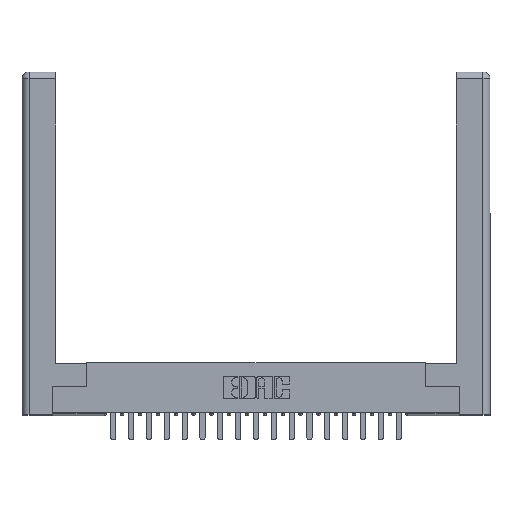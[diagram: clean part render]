
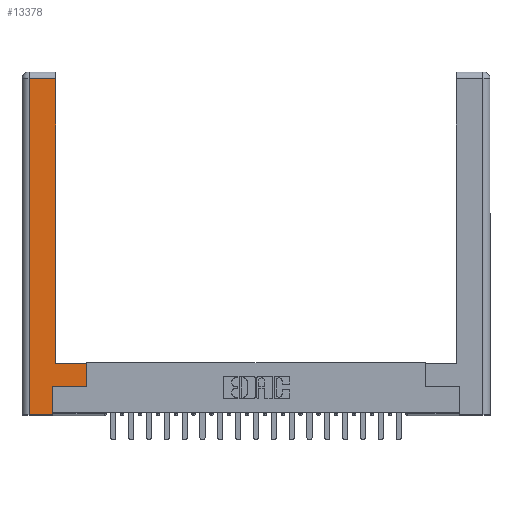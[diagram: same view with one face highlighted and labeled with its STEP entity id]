
A CAD part, top view. The second image highlights one B-rep face of the part: STEP entity #13378.
In plain terms, the highlighted planar face has unit normal (0, 0, 1).
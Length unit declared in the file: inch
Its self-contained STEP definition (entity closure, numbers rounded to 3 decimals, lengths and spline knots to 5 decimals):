
#65 = LINE ( 'NONE', #10941, #19154 ) ;
#107 = VECTOR ( 'NONE', #4367, 39.37008 ) ;
#343 = LINE ( 'NONE', #12468, #22065 ) ;
#572 = DIRECTION ( 'NONE',  ( -1., 0., 0. ) ) ;
#976 = CARTESIAN_POINT ( 'NONE',  ( 0.565, 0.245, 0. ) ) ;
#1050 = ORIENTED_EDGE ( 'NONE', *, *, #21979, .T. ) ;
#1167 = VECTOR ( 'NONE', #1383, 39.37008 ) ;
#1187 = LINE ( 'NONE', #21142, #4962 ) ;
#1383 = DIRECTION ( 'NONE',  ( 1., 0., 0. ) ) ;
#1439 = DIRECTION ( 'NONE',  ( 1., 0., 0. ) ) ;
#1939 = PLANE ( 'NONE',  #17478 ) ;
#2504 = CARTESIAN_POINT ( 'NONE',  ( 0.295, 0.45, 0. ) ) ;
#2881 = LINE ( 'NONE', #6658, #11604 ) ;
#2924 = DIRECTION ( 'NONE',  ( 0., 1., 0. ) ) ;
#3566 = ORIENTED_EDGE ( 'NONE', *, *, #14020, .T. ) ;
#4140 = LINE ( 'NONE', #15375, #20902 ) ;
#4367 = DIRECTION ( 'NONE',  ( 0., 1., 0. ) ) ;
#4962 = VECTOR ( 'NONE', #10049, 39.37008 ) ;
#5675 = VERTEX_POINT ( 'NONE', #2504 ) ;
#6290 = ORIENTED_EDGE ( 'NONE', *, *, #6470, .T. ) ;
#6310 = CARTESIAN_POINT ( 'NONE',  ( 0.295, 3., 0. ) ) ;
#6318 = CARTESIAN_POINT ( 'NONE',  ( 0.295, 2.94, 0. ) ) ;
#6350 = VERTEX_POINT ( 'NONE', #6318 ) ;
#6398 = EDGE_CURVE ( 'NONE', #6350, #15645, #4140, .T. ) ;
#6470 = EDGE_CURVE ( 'NONE', #15645, #20443, #65, .T. ) ;
#6608 = LINE ( 'NONE', #12666, #12117 ) ;
#6658 = CARTESIAN_POINT ( 'NONE',  ( 0.565, 0.45, 0. ) ) ;
#7301 = DIRECTION ( 'NONE',  ( 0., -1., 0. ) ) ;
#8088 = ORIENTED_EDGE ( 'NONE', *, *, #8609, .T. ) ;
#8609 = EDGE_CURVE ( 'NONE', #12126, #16049, #2881, .T. ) ;
#9026 = DIRECTION ( 'NONE',  ( 0., 1., 0. ) ) ;
#9556 = DIRECTION ( 'NONE',  ( 0., 0., -1. ) ) ;
#10049 = DIRECTION ( 'NONE',  ( -1., 0., 0. ) ) ;
#10516 = LINE ( 'NONE', #6310, #107 ) ;
#10620 = CARTESIAN_POINT ( 'NONE',  ( 0.565, 0.245, 0. ) ) ;
#10941 = CARTESIAN_POINT ( 'NONE',  ( 0.0615, 0., 0. ) ) ;
#11268 = DIRECTION ( 'NONE',  ( -1., 0., 0. ) ) ;
#11604 = VECTOR ( 'NONE', #2924, 39.37008 ) ;
#12117 = VECTOR ( 'NONE', #9026, 39.37008 ) ;
#12126 = VERTEX_POINT ( 'NONE', #976 ) ;
#12283 = EDGE_CURVE ( 'NONE', #13593, #12126, #14204, .T. ) ;
#12429 = FACE_OUTER_BOUND ( 'NONE', #15455, .T. ) ;
#12468 = CARTESIAN_POINT ( 'NONE',  ( 0.265, 0., 0. ) ) ;
#12492 = ORIENTED_EDGE ( 'NONE', *, *, #12283, .T. ) ;
#12666 = CARTESIAN_POINT ( 'NONE',  ( 0.265, 0.245, 0. ) ) ;
#13378 = ADVANCED_FACE ( 'NONE', ( #12429 ), #1939, .F. ) ;
#13593 = VERTEX_POINT ( 'NONE', #21556 ) ;
#14020 = EDGE_CURVE ( 'NONE', #23426, #13593, #6608, .T. ) ;
#14204 = LINE ( 'NONE', #10620, #1167 ) ;
#14820 = CARTESIAN_POINT ( 'NONE',  ( 0.565, 0.45, 0. ) ) ;
#14898 = ORIENTED_EDGE ( 'NONE', *, *, #6398, .T. ) ;
#15375 = CARTESIAN_POINT ( 'NONE',  ( 0.0615, 2.94, 0. ) ) ;
#15455 = EDGE_LOOP ( 'NONE', ( #1050, #14898, #6290, #18041, #3566, #12492, #8088, #17053 ) ) ;
#15645 = VERTEX_POINT ( 'NONE', #17046 ) ;
#16049 = VERTEX_POINT ( 'NONE', #14820 ) ;
#16658 = CARTESIAN_POINT ( 'NONE',  ( 0., 0., 0. ) ) ;
#17046 = CARTESIAN_POINT ( 'NONE',  ( 0.0615, 2.94, 0. ) ) ;
#17053 = ORIENTED_EDGE ( 'NONE', *, *, #17248, .T. ) ;
#17130 = EDGE_CURVE ( 'NONE', #20443, #23426, #343, .T. ) ;
#17248 = EDGE_CURVE ( 'NONE', #16049, #5675, #1187, .T. ) ;
#17478 = AXIS2_PLACEMENT_3D ( 'NONE', #16658, #9556, #11268 ) ;
#18041 = ORIENTED_EDGE ( 'NONE', *, *, #17130, .T. ) ;
#19154 = VECTOR ( 'NONE', #7301, 39.37008 ) ;
#19990 = CARTESIAN_POINT ( 'NONE',  ( 0.0615, 0., 0. ) ) ;
#20443 = VERTEX_POINT ( 'NONE', #19990 ) ;
#20902 = VECTOR ( 'NONE', #572, 39.37008 ) ;
#21142 = CARTESIAN_POINT ( 'NONE',  ( 0.295, 0.45, 0. ) ) ;
#21556 = CARTESIAN_POINT ( 'NONE',  ( 0.265, 0.245, 0. ) ) ;
#21979 = EDGE_CURVE ( 'NONE', #5675, #6350, #10516, .T. ) ;
#22065 = VECTOR ( 'NONE', #1439, 39.37008 ) ;
#22407 = CARTESIAN_POINT ( 'NONE',  ( 0.265, 0., 0. ) ) ;
#23426 = VERTEX_POINT ( 'NONE', #22407 ) ;
